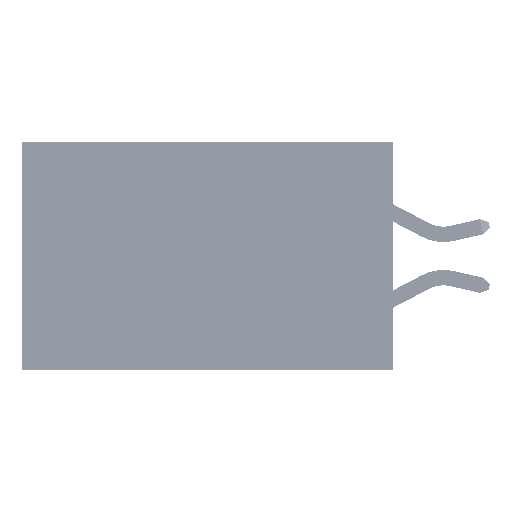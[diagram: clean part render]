
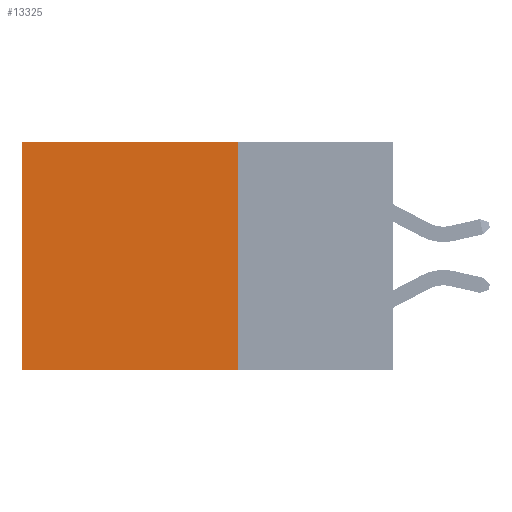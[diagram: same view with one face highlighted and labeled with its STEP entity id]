
A CAD part, left-side view. The second image highlights one B-rep face of the part: STEP entity #13325.
In plain terms, the highlighted planar face has unit normal (-1, 0, 0).
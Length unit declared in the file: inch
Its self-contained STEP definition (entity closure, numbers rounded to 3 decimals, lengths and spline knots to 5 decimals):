
#123 = CARTESIAN_POINT ( 'NONE',  ( 0.2875, 0.25, -0.37 ) ) ;
#1848 = AXIS2_PLACEMENT_3D ( 'NONE', #25148, #8894, #37420 ) ;
#2312 = ORIENTED_EDGE ( 'NONE', *, *, #46087, .F. ) ;
#2478 = VERTEX_POINT ( 'NONE', #23453 ) ;
#3823 = EDGE_LOOP ( 'NONE', ( #19731, #2312, #24151, #28165 ) ) ;
#4587 = VERTEX_POINT ( 'NONE', #123 ) ;
#8894 = DIRECTION ( 'NONE',  ( 1., 0., 0. ) ) ;
#10131 = LINE ( 'NONE', #39671, #42580 ) ;
#10557 = CARTESIAN_POINT ( 'NONE',  ( 0.2875, 0.6, 0. ) ) ;
#11872 = VERTEX_POINT ( 'NONE', #40534 ) ;
#13325 = ADVANCED_FACE ( 'NONE', ( #49747 ), #15952, .F. ) ;
#15952 = PLANE ( 'NONE',  #1848 ) ;
#16698 = EDGE_CURVE ( 'NONE', #29105, #2478, #35011, .T. ) ;
#17294 = VECTOR ( 'NONE', #28434, 39.37008 ) ;
#19731 = ORIENTED_EDGE ( 'NONE', *, *, #16698, .T. ) ;
#20188 = EDGE_CURVE ( 'NONE', #11872, #4587, #46818, .T. ) ;
#20467 = EDGE_CURVE ( 'NONE', #11872, #29105, #10131, .T. ) ;
#23453 = CARTESIAN_POINT ( 'NONE',  ( 0.2875, 0.6, -0.37 ) ) ;
#24145 = VECTOR ( 'NONE', #28802, 39.37008 ) ;
#24151 = ORIENTED_EDGE ( 'NONE', *, *, #20188, .F. ) ;
#25148 = CARTESIAN_POINT ( 'NONE',  ( 0.2875, 0.25, 0. ) ) ;
#28165 = ORIENTED_EDGE ( 'NONE', *, *, #20467, .T. ) ;
#28207 = LINE ( 'NONE', #48540, #17294 ) ;
#28434 = DIRECTION ( 'NONE',  ( 0., 1., 0. ) ) ;
#28802 = DIRECTION ( 'NONE',  ( 0., 0., -1. ) ) ;
#29105 = VERTEX_POINT ( 'NONE', #10557 ) ;
#32721 = CARTESIAN_POINT ( 'NONE',  ( 0.2875, 0.6, 0. ) ) ;
#33770 = VECTOR ( 'NONE', #34039, 39.37008 ) ;
#33863 = CARTESIAN_POINT ( 'NONE',  ( 0.2875, 0.25, 0. ) ) ;
#34039 = DIRECTION ( 'NONE',  ( 0., 0., -1. ) ) ;
#35011 = LINE ( 'NONE', #32721, #24145 ) ;
#37420 = DIRECTION ( 'NONE',  ( 0., 0., -1. ) ) ;
#39671 = CARTESIAN_POINT ( 'NONE',  ( 0.2875, 0.25, 0. ) ) ;
#40534 = CARTESIAN_POINT ( 'NONE',  ( 0.2875, 0.25, 0. ) ) ;
#42580 = VECTOR ( 'NONE', #43700, 39.37008 ) ;
#43700 = DIRECTION ( 'NONE',  ( 0., 1., 0. ) ) ;
#46087 = EDGE_CURVE ( 'NONE', #4587, #2478, #28207, .T. ) ;
#46818 = LINE ( 'NONE', #33863, #33770 ) ;
#48540 = CARTESIAN_POINT ( 'NONE',  ( 0.2875, 0.25, -0.37 ) ) ;
#49747 = FACE_OUTER_BOUND ( 'NONE', #3823, .T. ) ;
